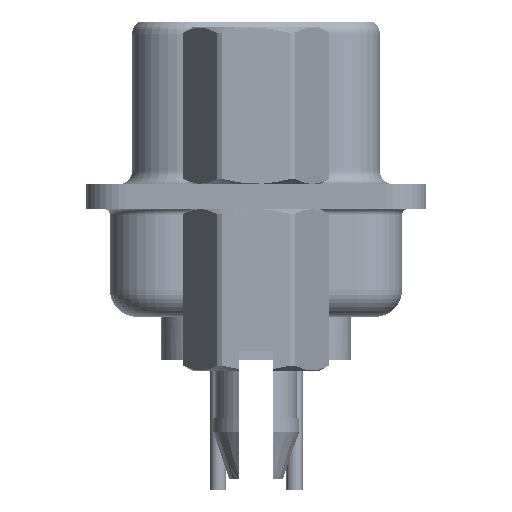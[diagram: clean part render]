
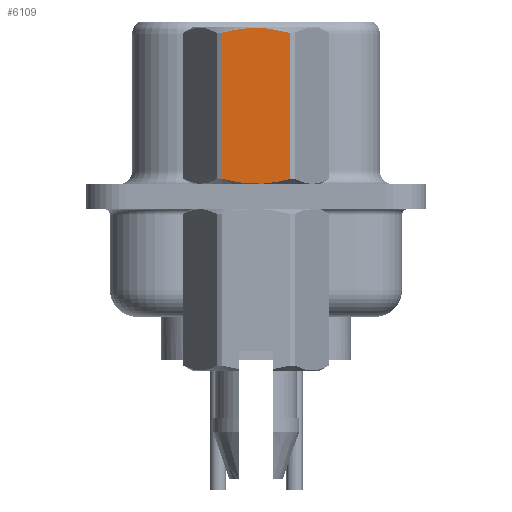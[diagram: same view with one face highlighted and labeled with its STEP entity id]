
A CAD part, left-side view. The second image highlights one B-rep face of the part: STEP entity #6109.
In plain terms, the highlighted planar face has unit normal (-1, 0, 0).
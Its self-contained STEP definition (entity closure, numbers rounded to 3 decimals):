
#14 = CARTESIAN_POINT ( 'NONE',  ( -2.381, 1.065, 6.104 ) ) ;
#353 = EDGE_CURVE ( 'NONE', #26807, #35251, #35387, .T. ) ;
#524 = DIRECTION ( 'NONE',  ( -1., 0., 0. ) ) ;
#1562 = DIRECTION ( 'NONE',  ( 0., 0., 1. ) ) ;
#1883 = AXIS2_PLACEMENT_3D ( 'NONE', #6456, #524, #11438 ) ;
#2196 = CARTESIAN_POINT ( 'NONE',  ( -2.381, -1.273, 0.652 ) ) ;
#3397 = ORIENTED_EDGE ( 'NONE', *, *, #28427, .T. ) ;
#3399 = VERTEX_POINT ( 'NONE', #2196 ) ;
#4604 = EDGE_CURVE ( 'NONE', #34830, #26807, #22893, .T. ) ;
#4862 = CARTESIAN_POINT ( 'NONE',  ( -2.381, 0.215, 6.232 ) ) ;
#5889 = CARTESIAN_POINT ( 'NONE',  ( -2.381, 0.428, 0.485 ) ) ;
#5912 = FACE_OUTER_BOUND ( 'NONE', #22421, .T. ) ;
#6109 = ADVANCED_FACE ( 'NONE', ( #5912 ), #16824, .T. ) ;
#6456 = CARTESIAN_POINT ( 'NONE',  ( -2.381, 1.375, -3.75 ) ) ;
#7273 = LINE ( 'NONE', #25950, #21002 ) ;
#9277 = CARTESIAN_POINT ( 'NONE',  ( -2.381, -1.273, 0.652 ) ) ;
#10668 = ORIENTED_EDGE ( 'NONE', *, *, #4604, .T. ) ;
#11438 = DIRECTION ( 'NONE',  ( 0., -1., 0. ) ) ;
#12673 = EDGE_CURVE ( 'NONE', #3399, #34830, #7273, .T. ) ;
#13257 = CARTESIAN_POINT ( 'NONE',  ( -2.381, -1.066, 6.104 ) ) ;
#14300 = CARTESIAN_POINT ( 'NONE',  ( -2.381, -0.858, 0.55 ) ) ;
#16801 = CARTESIAN_POINT ( 'NONE',  ( -2.381, 0.853, 0.549 ) ) ;
#16824 = PLANE ( 'NONE',  #1883 ) ;
#16986 = CARTESIAN_POINT ( 'NONE',  ( -2.381, -0.215, 0.468 ) ) ;
#17528 = CARTESIAN_POINT ( 'NONE',  ( -2.381, 1.273, 0.652 ) ) ;
#18465 = CARTESIAN_POINT ( 'NONE',  ( -2.381, -0.858, 6.15 ) ) ;
#18516 = CARTESIAN_POINT ( 'NONE',  ( -2.381, 1.273, 3.792 ) ) ;
#18996 = CARTESIAN_POINT ( 'NONE',  ( -2.381, -0.432, 6.215 ) ) ;
#20587 = CARTESIAN_POINT ( 'NONE',  ( -2.381, 1.273, 0.652 ) ) ;
#21002 = VECTOR ( 'NONE', #1562, 1000. ) ;
#22421 = EDGE_LOOP ( 'NONE', ( #3397, #28370, #10668, #34329 ) ) ;
#22539 = CARTESIAN_POINT ( 'NONE',  ( -2.381, 0.215, 0.468 ) ) ;
#22893 = B_SPLINE_CURVE_WITH_KNOTS ( 'NONE', 3,
 ( #32096, #13257, #18465, #18996, #29403, #4862, #26887, #26716, #14, #24021 ),
 .UNSPECIFIED., .F., .F.,
 ( 4, 2, 2, 2, 4 ),
 ( 0.001, 0.002, 0.002, 0.003, 0.004 ),
 .UNSPECIFIED. ) ;
#22903 = CARTESIAN_POINT ( 'NONE',  ( -2.381, 1.065, 0.596 ) ) ;
#23492 = CARTESIAN_POINT ( 'NONE',  ( -2.381, -1.273, 6.048 ) ) ;
#23759 = CARTESIAN_POINT ( 'NONE',  ( -2.381, 1.273, 6.048 ) ) ;
#24021 = CARTESIAN_POINT ( 'NONE',  ( -2.381, 1.273, 6.048 ) ) ;
#25142 = B_SPLINE_CURVE_WITH_KNOTS ( 'NONE', 3,
 ( #17528, #22903, #16801, #5889, #22539, #16986, #27736, #14300, #30612, #9277 ),
 .UNSPECIFIED., .F., .F.,
 ( 4, 2, 2, 2, 4 ),
 ( 0.003, 0.003, 0.004, 0.004, 0.005 ),
 .UNSPECIFIED. ) ;
#25950 = CARTESIAN_POINT ( 'NONE',  ( -2.381, -1.273, 3.792 ) ) ;
#26716 = CARTESIAN_POINT ( 'NONE',  ( -2.381, 0.853, 6.151 ) ) ;
#26807 = VERTEX_POINT ( 'NONE', #23759 ) ;
#26887 = CARTESIAN_POINT ( 'NONE',  ( -2.381, 0.428, 6.215 ) ) ;
#27736 = CARTESIAN_POINT ( 'NONE',  ( -2.381, -0.432, 0.485 ) ) ;
#28370 = ORIENTED_EDGE ( 'NONE', *, *, #12673, .T. ) ;
#28427 = EDGE_CURVE ( 'NONE', #35251, #3399, #25142, .T. ) ;
#29403 = CARTESIAN_POINT ( 'NONE',  ( -2.381, -0.215, 6.232 ) ) ;
#30339 = VECTOR ( 'NONE', #32158, 1000. ) ;
#30612 = CARTESIAN_POINT ( 'NONE',  ( -2.381, -1.066, 0.596 ) ) ;
#32096 = CARTESIAN_POINT ( 'NONE',  ( -2.381, -1.273, 6.048 ) ) ;
#32158 = DIRECTION ( 'NONE',  ( 0., 0., -1. ) ) ;
#34329 = ORIENTED_EDGE ( 'NONE', *, *, #353, .T. ) ;
#34830 = VERTEX_POINT ( 'NONE', #23492 ) ;
#35251 = VERTEX_POINT ( 'NONE', #20587 ) ;
#35387 = LINE ( 'NONE', #18516, #30339 ) ;
